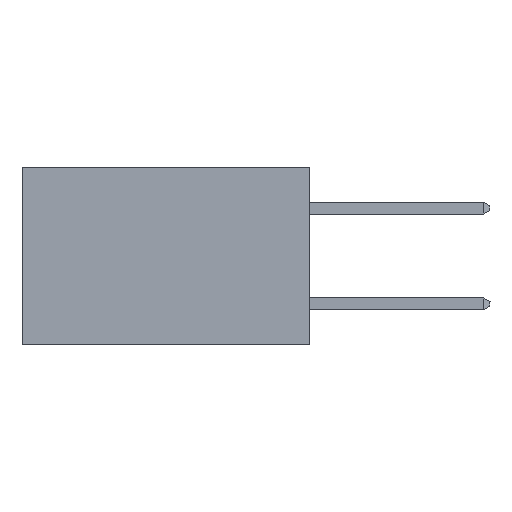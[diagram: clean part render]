
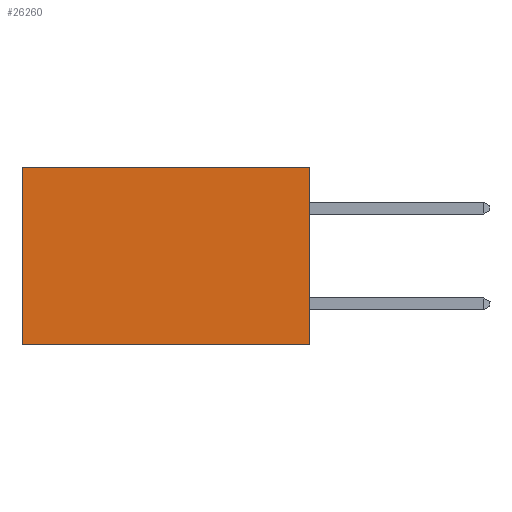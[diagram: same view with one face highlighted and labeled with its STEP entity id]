
A CAD part, left-side view. The second image highlights one B-rep face of the part: STEP entity #26260.
In plain terms, the highlighted planar face has unit normal (-1, 0, 0).
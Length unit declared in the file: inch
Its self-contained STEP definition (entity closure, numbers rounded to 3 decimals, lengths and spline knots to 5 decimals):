
#1907 = VECTOR ( 'NONE', #37628, 39.37008 ) ;
#2247 = DIRECTION ( 'NONE',  ( 0., 0., -1. ) ) ;
#2734 = AXIS2_PLACEMENT_3D ( 'NONE', #12240, #31707, #2247 ) ;
#10347 = CARTESIAN_POINT ( 'NONE',  ( 0.2875, 0.6, -0.37 ) ) ;
#10598 = LINE ( 'NONE', #14715, #1907 ) ;
#10735 = VERTEX_POINT ( 'NONE', #10347 ) ;
#11102 = VECTOR ( 'NONE', #41569, 39.37008 ) ;
#12240 = CARTESIAN_POINT ( 'NONE',  ( 0.2875, 0., 0. ) ) ;
#14715 = CARTESIAN_POINT ( 'NONE',  ( 0.2875, 0.6, 0. ) ) ;
#16076 = EDGE_LOOP ( 'NONE', ( #24090, #30934, #42130, #39230 ) ) ;
#17017 = VECTOR ( 'NONE', #22028, 39.37008 ) ;
#17793 = CARTESIAN_POINT ( 'NONE',  ( 0.2875, 0., 0. ) ) ;
#18078 = DIRECTION ( 'NONE',  ( 0., 0., -1. ) ) ;
#18469 = VERTEX_POINT ( 'NONE', #19926 ) ;
#19926 = CARTESIAN_POINT ( 'NONE',  ( 0.2875, 0., 0. ) ) ;
#22028 = DIRECTION ( 'NONE',  ( 0., 1., 0. ) ) ;
#23987 = CARTESIAN_POINT ( 'NONE',  ( 0.2875, 0.6, 0. ) ) ;
#24090 = ORIENTED_EDGE ( 'NONE', *, *, #31240, .T. ) ;
#25993 = VECTOR ( 'NONE', #18078, 39.37008 ) ;
#26260 = ADVANCED_FACE ( 'NONE', ( #36737 ), #31846, .F. ) ;
#29090 = VERTEX_POINT ( 'NONE', #30646 ) ;
#30376 = EDGE_CURVE ( 'NONE', #18469, #29090, #34729, .T. ) ;
#30646 = CARTESIAN_POINT ( 'NONE',  ( 0.2875, 0., -0.37 ) ) ;
#30862 = LINE ( 'NONE', #41466, #17017 ) ;
#30934 = ORIENTED_EDGE ( 'NONE', *, *, #38021, .F. ) ;
#31240 = EDGE_CURVE ( 'NONE', #42396, #10735, #10598, .T. ) ;
#31707 = DIRECTION ( 'NONE',  ( 1., 0., 0. ) ) ;
#31846 = PLANE ( 'NONE',  #2734 ) ;
#33658 = LINE ( 'NONE', #41853, #11102 ) ;
#34729 = LINE ( 'NONE', #17793, #25993 ) ;
#36737 = FACE_OUTER_BOUND ( 'NONE', #16076, .T. ) ;
#37628 = DIRECTION ( 'NONE',  ( 0., 0., -1. ) ) ;
#38021 = EDGE_CURVE ( 'NONE', #29090, #10735, #30862, .T. ) ;
#39230 = ORIENTED_EDGE ( 'NONE', *, *, #41039, .T. ) ;
#41039 = EDGE_CURVE ( 'NONE', #18469, #42396, #33658, .T. ) ;
#41466 = CARTESIAN_POINT ( 'NONE',  ( 0.2875, 0., -0.37 ) ) ;
#41569 = DIRECTION ( 'NONE',  ( 0., 1., 0. ) ) ;
#41853 = CARTESIAN_POINT ( 'NONE',  ( 0.2875, 0., 0. ) ) ;
#42130 = ORIENTED_EDGE ( 'NONE', *, *, #30376, .F. ) ;
#42396 = VERTEX_POINT ( 'NONE', #23987 ) ;
